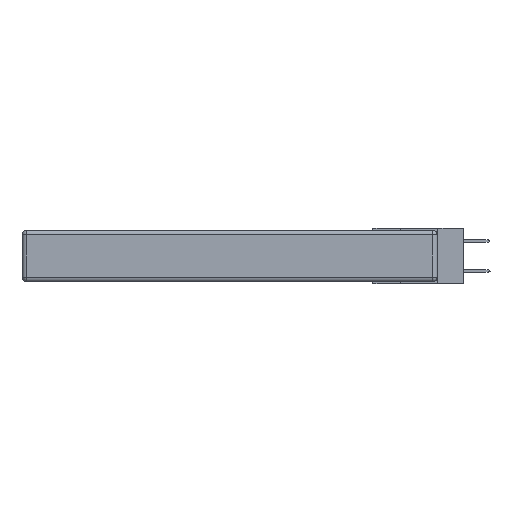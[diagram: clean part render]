
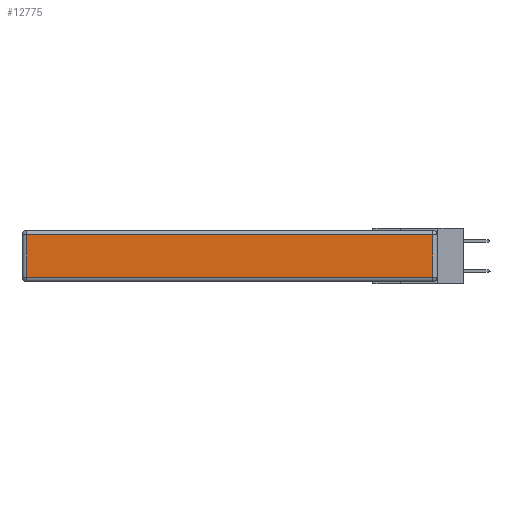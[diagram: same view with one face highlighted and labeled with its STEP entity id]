
A CAD part, left-side view. The second image highlights one B-rep face of the part: STEP entity #12775.
In plain terms, the highlighted planar face has unit normal (-1, 0, 0).
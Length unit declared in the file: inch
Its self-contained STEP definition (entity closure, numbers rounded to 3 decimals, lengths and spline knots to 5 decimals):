
#532 = FACE_OUTER_BOUND ( 'NONE', #12013, .T. ) ;
#958 = CARTESIAN_POINT ( 'NONE',  ( 0., 2.72, -0.343 ) ) ;
#1921 = VERTEX_POINT ( 'NONE', #29396 ) ;
#2042 = EDGE_CURVE ( 'NONE', #4420, #1921, #6683, .T. ) ;
#2300 = VERTEX_POINT ( 'NONE', #13308 ) ;
#3067 = AXIS2_PLACEMENT_3D ( 'NONE', #25274, #18095, #5436 ) ;
#3882 = ORIENTED_EDGE ( 'NONE', *, *, #25057, .T. ) ;
#4420 = VERTEX_POINT ( 'NONE', #5472 ) ;
#4545 = ORIENTED_EDGE ( 'NONE', *, *, #2042, .T. ) ;
#5436 = DIRECTION ( 'NONE',  ( 0., 0., 1. ) ) ;
#5472 = CARTESIAN_POINT ( 'NONE',  ( 0., 2.72, -0.03 ) ) ;
#6683 = LINE ( 'NONE', #958, #26278 ) ;
#7781 = CARTESIAN_POINT ( 'NONE',  ( 0., 0.03, -0.03 ) ) ;
#8733 = LINE ( 'NONE', #14827, #19400 ) ;
#9265 = DIRECTION ( 'NONE',  ( 0., 0., 1. ) ) ;
#10005 = DIRECTION ( 'NONE',  ( 0., -1., 0. ) ) ;
#11189 = EDGE_CURVE ( 'NONE', #12159, #4420, #22112, .T. ) ;
#11791 = VECTOR ( 'NONE', #27656, 39.37008 ) ;
#12013 = EDGE_LOOP ( 'NONE', ( #20141, #3882, #13767, #4545 ) ) ;
#12159 = VERTEX_POINT ( 'NONE', #7781 ) ;
#12775 = ADVANCED_FACE ( 'NONE', ( #532 ), #17988, .T. ) ;
#13308 = CARTESIAN_POINT ( 'NONE',  ( 0., 0.03, -0.313 ) ) ;
#13767 = ORIENTED_EDGE ( 'NONE', *, *, #11189, .T. ) ;
#14827 = CARTESIAN_POINT ( 'NONE',  ( 0., 0., -0.313 ) ) ;
#17988 = PLANE ( 'NONE',  #3067 ) ;
#18095 = DIRECTION ( 'NONE',  ( -1., 0., 0. ) ) ;
#18456 = CARTESIAN_POINT ( 'NONE',  ( 0., 0.03, -0.343 ) ) ;
#19400 = VECTOR ( 'NONE', #10005, 39.37008 ) ;
#20141 = ORIENTED_EDGE ( 'NONE', *, *, #21569, .T. ) ;
#20143 = VECTOR ( 'NONE', #9265, 39.37008 ) ;
#21569 = EDGE_CURVE ( 'NONE', #1921, #2300, #8733, .T. ) ;
#22112 = LINE ( 'NONE', #25728, #11791 ) ;
#25057 = EDGE_CURVE ( 'NONE', #2300, #12159, #25531, .T. ) ;
#25274 = CARTESIAN_POINT ( 'NONE',  ( 0., 0., -0.343 ) ) ;
#25531 = LINE ( 'NONE', #18456, #20143 ) ;
#25728 = CARTESIAN_POINT ( 'NONE',  ( 0., 2.75, -0.03 ) ) ;
#26278 = VECTOR ( 'NONE', #30562, 39.37008 ) ;
#27656 = DIRECTION ( 'NONE',  ( 0., 1., 0. ) ) ;
#29396 = CARTESIAN_POINT ( 'NONE',  ( 0., 2.72, -0.313 ) ) ;
#30562 = DIRECTION ( 'NONE',  ( 0., 0., -1. ) ) ;
